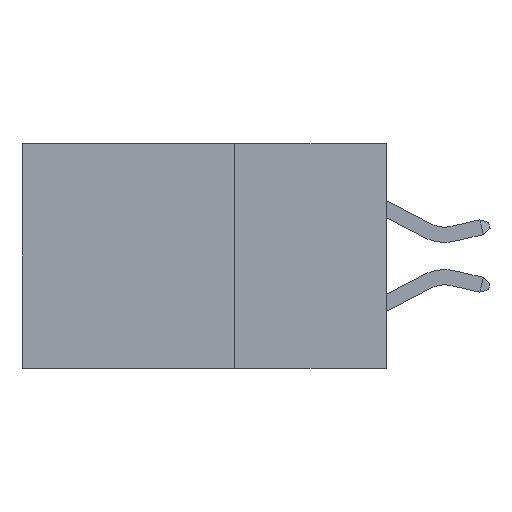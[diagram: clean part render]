
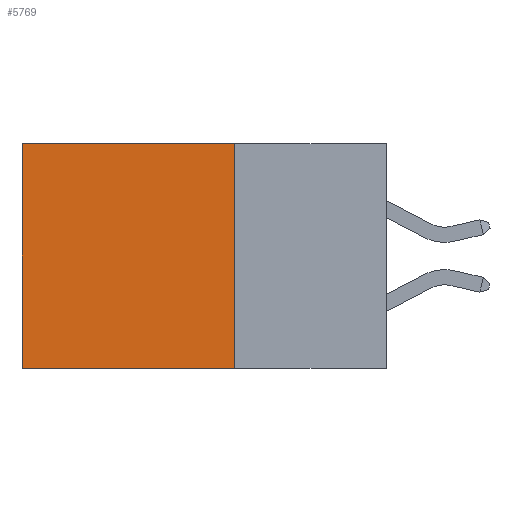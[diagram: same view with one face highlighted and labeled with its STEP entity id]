
A CAD part, left-side view. The second image highlights one B-rep face of the part: STEP entity #5769.
In plain terms, the highlighted planar face has unit normal (-1, 0, 0).
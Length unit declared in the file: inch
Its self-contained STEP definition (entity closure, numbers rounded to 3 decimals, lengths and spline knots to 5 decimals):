
#331 = CARTESIAN_POINT ( 'NONE',  ( 0.298, 0.6, -0.37 ) ) ;
#1179 = CARTESIAN_POINT ( 'NONE',  ( 0.298, 0.25, 0. ) ) ;
#1550 = EDGE_CURVE ( 'NONE', #14897, #7537, #18572, .T. ) ;
#3082 = VECTOR ( 'NONE', #3576, 39.37008 ) ;
#3548 = VECTOR ( 'NONE', #6745, 39.37008 ) ;
#3576 = DIRECTION ( 'NONE',  ( 0., 0., -1. ) ) ;
#5703 = CARTESIAN_POINT ( 'NONE',  ( 0.298, 0.25, 0. ) ) ;
#5769 = ADVANCED_FACE ( 'NONE', ( #17820 ), #7459, .F. ) ;
#5940 = ORIENTED_EDGE ( 'NONE', *, *, #6762, .F. ) ;
#6321 = ORIENTED_EDGE ( 'NONE', *, *, #14879, .T. ) ;
#6574 = LINE ( 'NONE', #10291, #16579 ) ;
#6745 = DIRECTION ( 'NONE',  ( 0., 1., 0. ) ) ;
#6762 = EDGE_CURVE ( 'NONE', #16280, #10084, #6574, .T. ) ;
#6919 = LINE ( 'NONE', #16757, #3082 ) ;
#7373 = CARTESIAN_POINT ( 'NONE',  ( 0.298, 0.25, 0. ) ) ;
#7459 = PLANE ( 'NONE',  #22510 ) ;
#7537 = VERTEX_POINT ( 'NONE', #16466 ) ;
#9156 = LINE ( 'NONE', #19300, #18560 ) ;
#9975 = DIRECTION ( 'NONE',  ( 0., 0., -1. ) ) ;
#10084 = VERTEX_POINT ( 'NONE', #331 ) ;
#10291 = CARTESIAN_POINT ( 'NONE',  ( 0.298, 0.25, -0.37 ) ) ;
#11237 = EDGE_LOOP ( 'NONE', ( #6321, #5940, #19751, #21146 ) ) ;
#11439 = DIRECTION ( 'NONE',  ( 0., 0., -1. ) ) ;
#14879 = EDGE_CURVE ( 'NONE', #7537, #10084, #6919, .T. ) ;
#14897 = VERTEX_POINT ( 'NONE', #7373 ) ;
#16280 = VERTEX_POINT ( 'NONE', #20917 ) ;
#16466 = CARTESIAN_POINT ( 'NONE',  ( 0.298, 0.6, 0. ) ) ;
#16579 = VECTOR ( 'NONE', #23340, 39.37008 ) ;
#16757 = CARTESIAN_POINT ( 'NONE',  ( 0.298, 0.6, 0. ) ) ;
#17820 = FACE_OUTER_BOUND ( 'NONE', #11237, .T. ) ;
#18560 = VECTOR ( 'NONE', #9975, 39.37008 ) ;
#18572 = LINE ( 'NONE', #1179, #3548 ) ;
#19300 = CARTESIAN_POINT ( 'NONE',  ( 0.298, 0.25, 0. ) ) ;
#19751 = ORIENTED_EDGE ( 'NONE', *, *, #21499, .F. ) ;
#20917 = CARTESIAN_POINT ( 'NONE',  ( 0.298, 0.25, -0.37 ) ) ;
#21146 = ORIENTED_EDGE ( 'NONE', *, *, #1550, .T. ) ;
#21499 = EDGE_CURVE ( 'NONE', #14897, #16280, #9156, .T. ) ;
#22510 = AXIS2_PLACEMENT_3D ( 'NONE', #5703, #22612, #11439 ) ;
#22612 = DIRECTION ( 'NONE',  ( 1., 0., 0. ) ) ;
#23340 = DIRECTION ( 'NONE',  ( 0., 1., 0. ) ) ;
